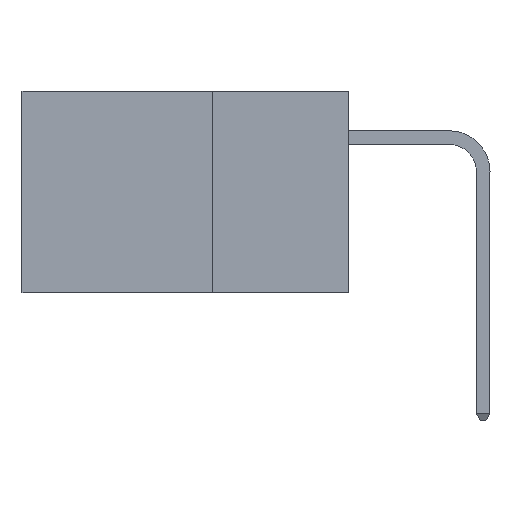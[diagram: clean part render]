
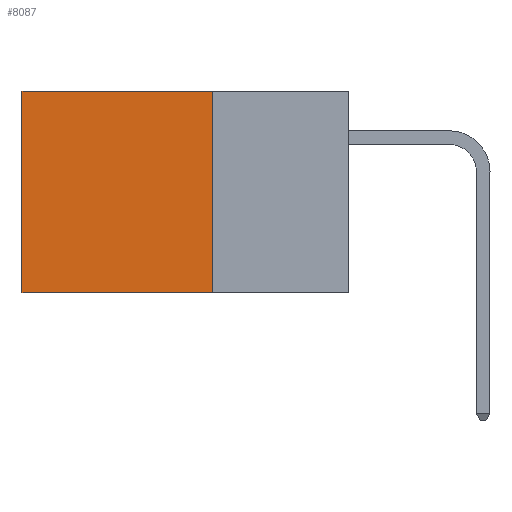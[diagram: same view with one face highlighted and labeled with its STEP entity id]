
A CAD part, left-side view. The second image highlights one B-rep face of the part: STEP entity #8087.
In plain terms, the highlighted planar face has unit normal (-1, 0, 0).
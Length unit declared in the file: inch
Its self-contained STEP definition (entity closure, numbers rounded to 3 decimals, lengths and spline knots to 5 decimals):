
#601 = AXIS2_PLACEMENT_3D ( 'NONE', #35956, #18803, #1318 ) ;
#1318 = DIRECTION ( 'NONE',  ( 0., 0., -1. ) ) ;
#1600 = CARTESIAN_POINT ( 'NONE',  ( 0.2875, 0.25, 0. ) ) ;
#1702 = CARTESIAN_POINT ( 'NONE',  ( 0.2875, 0.25, 0. ) ) ;
#3197 = CARTESIAN_POINT ( 'NONE',  ( 0.2875, 0.25, -0.37 ) ) ;
#4497 = ORIENTED_EDGE ( 'NONE', *, *, #33724, .T. ) ;
#6053 = ORIENTED_EDGE ( 'NONE', *, *, #35476, .F. ) ;
#6308 = EDGE_CURVE ( 'NONE', #8841, #28479, #29673, .T. ) ;
#8087 = ADVANCED_FACE ( 'NONE', ( #12200 ), #33103, .F. ) ;
#8269 = LINE ( 'NONE', #3197, #23732 ) ;
#8452 = ORIENTED_EDGE ( 'NONE', *, *, #26807, .T. ) ;
#8841 = VERTEX_POINT ( 'NONE', #1600 ) ;
#11644 = ORIENTED_EDGE ( 'NONE', *, *, #6308, .F. ) ;
#12200 = FACE_OUTER_BOUND ( 'NONE', #21522, .T. ) ;
#13300 = VERTEX_POINT ( 'NONE', #27609 ) ;
#14259 = VECTOR ( 'NONE', #27851, 39.37008 ) ;
#17313 = DIRECTION ( 'NONE',  ( 0., 1., 0. ) ) ;
#18803 = DIRECTION ( 'NONE',  ( 1., 0., 0. ) ) ;
#19448 = LINE ( 'NONE', #35304, #26204 ) ;
#20254 = LINE ( 'NONE', #34517, #35503 ) ;
#21015 = DIRECTION ( 'NONE',  ( 0., 0., -1. ) ) ;
#21522 = EDGE_LOOP ( 'NONE', ( #8452, #6053, #11644, #4497 ) ) ;
#23554 = DIRECTION ( 'NONE',  ( 0., 1., 0. ) ) ;
#23732 = VECTOR ( 'NONE', #23554, 39.37008 ) ;
#24974 = VERTEX_POINT ( 'NONE', #36687 ) ;
#26204 = VECTOR ( 'NONE', #21015, 39.37008 ) ;
#26807 = EDGE_CURVE ( 'NONE', #13300, #24974, #19448, .T. ) ;
#27609 = CARTESIAN_POINT ( 'NONE',  ( 0.2875, 0.6, 0. ) ) ;
#27851 = DIRECTION ( 'NONE',  ( 0., 0., -1. ) ) ;
#28479 = VERTEX_POINT ( 'NONE', #34450 ) ;
#29673 = LINE ( 'NONE', #1702, #14259 ) ;
#33103 = PLANE ( 'NONE',  #601 ) ;
#33724 = EDGE_CURVE ( 'NONE', #8841, #13300, #20254, .T. ) ;
#34450 = CARTESIAN_POINT ( 'NONE',  ( 0.2875, 0.25, -0.37 ) ) ;
#34517 = CARTESIAN_POINT ( 'NONE',  ( 0.2875, 0.25, 0. ) ) ;
#35304 = CARTESIAN_POINT ( 'NONE',  ( 0.2875, 0.6, 0. ) ) ;
#35476 = EDGE_CURVE ( 'NONE', #28479, #24974, #8269, .T. ) ;
#35503 = VECTOR ( 'NONE', #17313, 39.37008 ) ;
#35956 = CARTESIAN_POINT ( 'NONE',  ( 0.2875, 0.25, 0. ) ) ;
#36687 = CARTESIAN_POINT ( 'NONE',  ( 0.2875, 0.6, -0.37 ) ) ;
